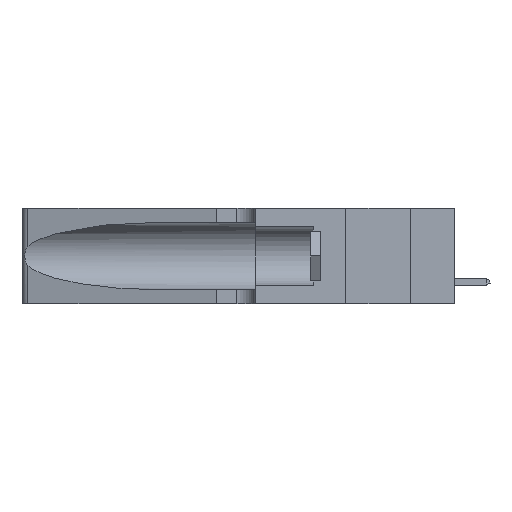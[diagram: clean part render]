
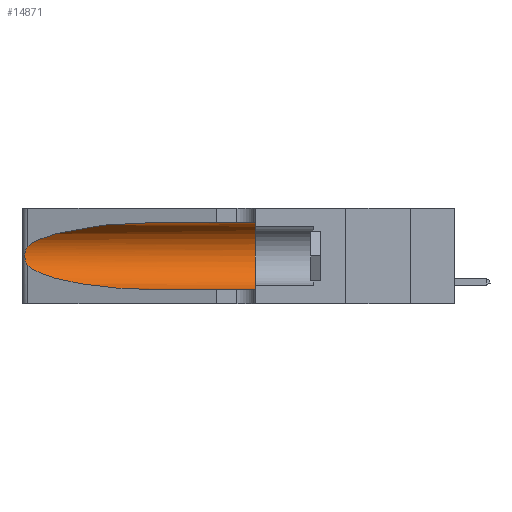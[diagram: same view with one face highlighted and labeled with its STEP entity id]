
A CAD part, left-side view. The second image highlights one B-rep face of the part: STEP entity #14871.
In plain terms, the highlighted cylindrical face has radius 3.308 mm (diameter 6.617 mm), a partial arc.
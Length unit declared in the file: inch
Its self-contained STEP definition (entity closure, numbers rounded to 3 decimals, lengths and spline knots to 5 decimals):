
#637 = CARTESIAN_POINT ( 'NONE',  ( 0.25555, 1.22993, 0.14849 ) ) ;
#1027 =( BOUNDED_CURVE ( )  B_SPLINE_CURVE ( 3, ( #27688, #10053, #6463, #20984 ),
 .UNSPECIFIED., .F., .T. ) 
 B_SPLINE_CURVE_WITH_KNOTS ( ( 4, 4 ),
 ( 1.5708, 2.84003 ),
 .UNSPECIFIED. ) 
 CURVE ( )  GEOMETRIC_REPRESENTATION_ITEM ( )  RATIONAL_B_SPLINE_CURVE ( ( 1., 0.87, 0.87, 1. ) ) 
 REPRESENTATION_ITEM ( '' )  );
#1666 =( BOUNDED_CURVE ( )  B_SPLINE_CURVE ( 3, ( #4702, #25908, #36882, #26228 ),
 .UNSPECIFIED., .F., .T. ) 
 B_SPLINE_CURVE_WITH_KNOTS ( ( 4, 4 ),
 ( 3.44316, 4.71239 ),
 .UNSPECIFIED. ) 
 CURVE ( )  GEOMETRIC_REPRESENTATION_ITEM ( )  RATIONAL_B_SPLINE_CURVE ( ( 1., 0.87, 0.87, 1. ) ) 
 REPRESENTATION_ITEM ( '' )  );
#4702 = CARTESIAN_POINT ( 'NONE',  ( 0.25487, 1.22718, 0.14631 ) ) ;
#4985 = CARTESIAN_POINT ( 'NONE',  ( 0.1305, 1.61858, 0.31525 ) ) ;
#5717 = ORIENTED_EDGE ( 'NONE', *, *, #27010, .F. ) ;
#5942 = LINE ( 'NONE', #4985, #27170 ) ;
#6116 = EDGE_CURVE ( 'NONE', #43782, #14728, #17729, .T. ) ;
#6463 = CARTESIAN_POINT ( 'NONE',  ( 0.2373, 1.15595, 0.28018 ) ) ;
#6967 = VERTEX_POINT ( 'NONE', #43248 ) ;
#7299 = CARTESIAN_POINT ( 'NONE',  ( 0.26075, 1.23896, 0.178 ) ) ;
#7321 = ORIENTED_EDGE ( 'NONE', *, *, #35940, .T. ) ;
#7771 = AXIS2_PLACEMENT_3D ( 'NONE', #41811, #42290, #45878 ) ;
#8717 = EDGE_LOOP ( 'NONE', ( #42581, #16312, #28831, #7321, #5717, #38731 ) ) ;
#9069 = AXIS2_PLACEMENT_3D ( 'NONE', #28986, #21953, #28843 ) ;
#9496 = EDGE_CURVE ( 'NONE', #19625, #45227, #5942, .T. ) ;
#10053 = CARTESIAN_POINT ( 'NONE',  ( 0.18966, 0.96281, 0.31525 ) ) ;
#10618 = CIRCLE ( 'NONE', #9069, 0.13025 ) ;
#14728 = VERTEX_POINT ( 'NONE', #40669 ) ;
#14871 = ADVANCED_FACE ( 'NONE', ( #41596 ), #22550, .F. ) ;
#16312 = ORIENTED_EDGE ( 'NONE', *, *, #6116, .T. ) ;
#17495 = CARTESIAN_POINT ( 'NONE',  ( 0.25639, 1.23184, 0.21858 ) ) ;
#17729 = B_SPLINE_CURVE_WITH_KNOTS ( 'NONE', 3,
 ( #42304, #45898, #17495, #24635, #18061, #36312, #39322, #7299, #18484, #25204, #21799, #18338, #637, #40671 ),
 .UNSPECIFIED., .F., .F.,
 ( 4, 2, 2, 2, 2, 2, 4 ),
 ( 0., 0.00027, 0.00053, 0.00107, 0.0016, 0.00187, 0.00214 ),
 .UNSPECIFIED. ) ;
#18061 = CARTESIAN_POINT ( 'NONE',  ( 0.25854, 1.2359, 0.20912 ) ) ;
#18338 = CARTESIAN_POINT ( 'NONE',  ( 0.25639, 1.23186, 0.15144 ) ) ;
#18484 = CARTESIAN_POINT ( 'NONE',  ( 0.26017, 1.23833, 0.17102 ) ) ;
#19178 = EDGE_CURVE ( 'NONE', #14728, #41024, #1666, .T. ) ;
#19215 = CARTESIAN_POINT ( 'NONE',  ( 0.25487, 1.22718, 0.22369 ) ) ;
#19625 = VERTEX_POINT ( 'NONE', #39926 ) ;
#19857 = CARTESIAN_POINT ( 'NONE',  ( 0.1305, 1.61858, 0.05475 ) ) ;
#20984 = CARTESIAN_POINT ( 'NONE',  ( 0.25487, 1.22718, 0.22369 ) ) ;
#21799 = CARTESIAN_POINT ( 'NONE',  ( 0.25789, 1.23486, 0.15765 ) ) ;
#21953 = DIRECTION ( 'NONE',  ( 0., 1., 0. ) ) ;
#22550 = CYLINDRICAL_SURFACE ( 'NONE', #7771, 0.13025 ) ;
#23947 = CARTESIAN_POINT ( 'NONE',  ( 0.1305, 0.35, 0.31525 ) ) ;
#24635 = CARTESIAN_POINT ( 'NONE',  ( 0.25787, 1.23484, 0.2124 ) ) ;
#25204 = CARTESIAN_POINT ( 'NONE',  ( 0.25856, 1.23593, 0.16098 ) ) ;
#25908 = CARTESIAN_POINT ( 'NONE',  ( 0.2373, 1.15595, 0.08982 ) ) ;
#26228 = CARTESIAN_POINT ( 'NONE',  ( 0.1305, 0.72297, 0.05475 ) ) ;
#27010 = EDGE_CURVE ( 'NONE', #45227, #6967, #10618, .T. ) ;
#27170 = VECTOR ( 'NONE', #30438, 39.37008 ) ;
#27688 = CARTESIAN_POINT ( 'NONE',  ( 0.1305, 0.72297, 0.31525 ) ) ;
#28831 = ORIENTED_EDGE ( 'NONE', *, *, #19178, .T. ) ;
#28843 = DIRECTION ( 'NONE',  ( 0., 0., 1. ) ) ;
#28986 = CARTESIAN_POINT ( 'NONE',  ( 0.1305, 0.35, 0.185 ) ) ;
#29013 = CARTESIAN_POINT ( 'NONE',  ( 0.1305, 0.72297, 0.05475 ) ) ;
#30438 = DIRECTION ( 'NONE',  ( 0., -1., 0. ) ) ;
#32862 = VECTOR ( 'NONE', #44842, 39.37008 ) ;
#35940 = EDGE_CURVE ( 'NONE', #41024, #6967, #40096, .T. ) ;
#36312 = CARTESIAN_POINT ( 'NONE',  ( 0.26018, 1.23835, 0.19895 ) ) ;
#36882 = CARTESIAN_POINT ( 'NONE',  ( 0.18966, 0.96281, 0.05475 ) ) ;
#38731 = ORIENTED_EDGE ( 'NONE', *, *, #9496, .F. ) ;
#39322 = CARTESIAN_POINT ( 'NONE',  ( 0.26075, 1.23896, 0.19203 ) ) ;
#39926 = CARTESIAN_POINT ( 'NONE',  ( 0.1305, 0.72297, 0.31525 ) ) ;
#40096 = LINE ( 'NONE', #19857, #32862 ) ;
#40669 = CARTESIAN_POINT ( 'NONE',  ( 0.25487, 1.22718, 0.14631 ) ) ;
#40671 = CARTESIAN_POINT ( 'NONE',  ( 0.25487, 1.22718, 0.14631 ) ) ;
#41024 = VERTEX_POINT ( 'NONE', #29013 ) ;
#41596 = FACE_OUTER_BOUND ( 'NONE', #8717, .T. ) ;
#41811 = CARTESIAN_POINT ( 'NONE',  ( 0.1305, 1.61858, 0.185 ) ) ;
#42290 = DIRECTION ( 'NONE',  ( 0., -1., 0. ) ) ;
#42304 = CARTESIAN_POINT ( 'NONE',  ( 0.25487, 1.22718, 0.22369 ) ) ;
#42581 = ORIENTED_EDGE ( 'NONE', *, *, #45761, .T. ) ;
#43248 = CARTESIAN_POINT ( 'NONE',  ( 0.1305, 0.35, 0.05475 ) ) ;
#43782 = VERTEX_POINT ( 'NONE', #19215 ) ;
#44842 = DIRECTION ( 'NONE',  ( 0., -1., 0. ) ) ;
#45227 = VERTEX_POINT ( 'NONE', #23947 ) ;
#45761 = EDGE_CURVE ( 'NONE', #19625, #43782, #1027, .T. ) ;
#45878 = DIRECTION ( 'NONE',  ( 0., 0., -1. ) ) ;
#45898 = CARTESIAN_POINT ( 'NONE',  ( 0.25555, 1.22994, 0.2215 ) ) ;
